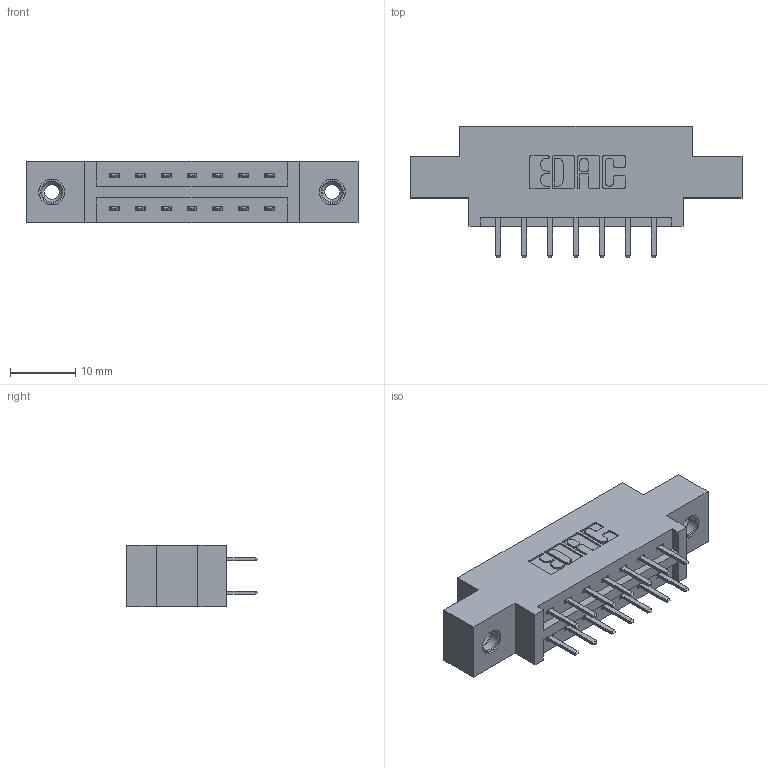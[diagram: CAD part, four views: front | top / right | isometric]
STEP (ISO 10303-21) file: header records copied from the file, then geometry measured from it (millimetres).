
FILE_DESCRIPTION (( 'STEP AP203' ), '1' );
FILE_NAME ('387-014-520-808.STEP', '2018-09-11T02:10:18', ( '' ), ( '' ), 'SwSTEP 2.0', 'SolidWorks 2016', '' );
FILE_SCHEMA (( 'CONFIG_CONTROL_DESIGN' ));
Length unit declared in the file: inch
Products named in the file (4): 345-292-001_345-293-120; 345-250-001_345-250-003-102; 387-014-520-808; 337 Part_0.170 Offset - 0.156 Dia-TI
Assembly tree (17 placements, depth 2):
  387-014-520-808
    337 Part_0.170 Offset - 0.156 Dia-TI
    345-292-001_345-293-120  x14
    345-250-001_345-250-003-102  x2
Bounding box: 50.75 x 20.02 x 9.4 mm (x, y, z)
Volume: 4752.3 mm3; surface area: 5146.7 mm2
Topology: 17 solids, 17 shells, 990 faces, 2825 edges, 1838 vertices
Faces by surface type: plane 666, cylinder 308, cone 12, torus 4
Entity records: 11386 total; most frequent: CARTESIAN_POINT 1941, ORIENTED_EDGE 1858, DIRECTION 1735, EDGE_CURVE 929, VECTOR 777, LINE 777, VERTEX_POINT 612, AXIS2_PLACEMENT_3D 479
